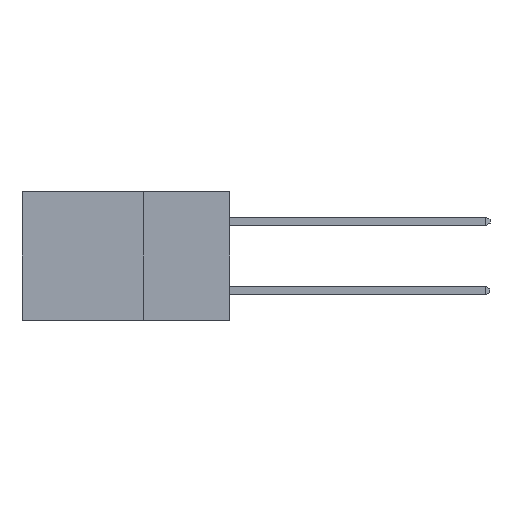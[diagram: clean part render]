
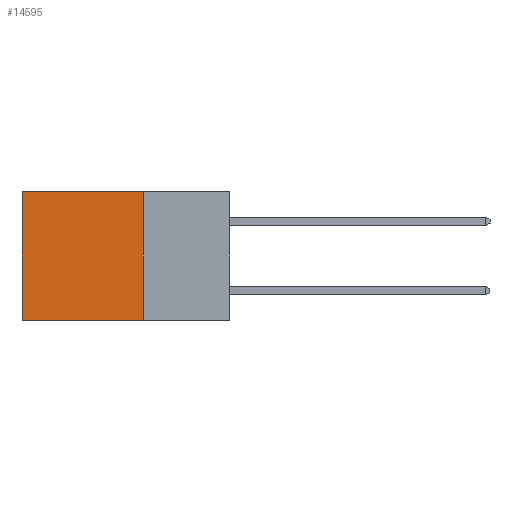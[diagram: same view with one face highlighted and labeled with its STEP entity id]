
A CAD part, left-side view. The second image highlights one B-rep face of the part: STEP entity #14595.
In plain terms, the highlighted planar face has unit normal (-1, 0, 0).
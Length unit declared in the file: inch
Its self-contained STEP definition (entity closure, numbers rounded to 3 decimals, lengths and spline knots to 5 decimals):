
#228 = EDGE_CURVE ( 'NONE', #10772, #3027, #12174, .T. ) ;
#235 = CARTESIAN_POINT ( 'NONE',  ( 0.298, 0.25, 0. ) ) ;
#548 = CARTESIAN_POINT ( 'NONE',  ( 0.298, 0.25, -0.37 ) ) ;
#969 = DIRECTION ( 'NONE',  ( 0., 0., -1. ) ) ;
#998 = EDGE_CURVE ( 'NONE', #12565, #10772, #10539, .T. ) ;
#1278 = LINE ( 'NONE', #548, #7105 ) ;
#1684 = CARTESIAN_POINT ( 'NONE',  ( 0.298, 0.6, 0. ) ) ;
#2713 = DIRECTION ( 'NONE',  ( 1., 0., 0. ) ) ;
#3027 = VERTEX_POINT ( 'NONE', #4455 ) ;
#3034 = CARTESIAN_POINT ( 'NONE',  ( 0.298, 0.6, 0. ) ) ;
#3266 = LINE ( 'NONE', #3469, #9835 ) ;
#3284 = ORIENTED_EDGE ( 'NONE', *, *, #228, .T. ) ;
#3469 = CARTESIAN_POINT ( 'NONE',  ( 0.298, 0.25, 0. ) ) ;
#4455 = CARTESIAN_POINT ( 'NONE',  ( 0.298, 0.6, -0.37 ) ) ;
#4891 = DIRECTION ( 'NONE',  ( 0., 1., 0. ) ) ;
#4924 = EDGE_LOOP ( 'NONE', ( #3284, #9268, #8479, #12929 ) ) ;
#5196 = DIRECTION ( 'NONE',  ( 0., 1., 0. ) ) ;
#6212 = PLANE ( 'NONE',  #14127 ) ;
#7105 = VECTOR ( 'NONE', #5196, 39.37008 ) ;
#7420 = VECTOR ( 'NONE', #4891, 39.37008 ) ;
#7896 = CARTESIAN_POINT ( 'NONE',  ( 0.298, 0.25, -0.37 ) ) ;
#8479 = ORIENTED_EDGE ( 'NONE', *, *, #14366, .F. ) ;
#8539 = DIRECTION ( 'NONE',  ( 0., 0., -1. ) ) ;
#9268 = ORIENTED_EDGE ( 'NONE', *, *, #12765, .F. ) ;
#9835 = VECTOR ( 'NONE', #11619, 39.37008 ) ;
#10539 = LINE ( 'NONE', #13811, #7420 ) ;
#10757 = CARTESIAN_POINT ( 'NONE',  ( 0.298, 0.25, 0. ) ) ;
#10772 = VERTEX_POINT ( 'NONE', #1684 ) ;
#11619 = DIRECTION ( 'NONE',  ( 0., 0., -1. ) ) ;
#11813 = VECTOR ( 'NONE', #969, 39.37008 ) ;
#12174 = LINE ( 'NONE', #3034, #11813 ) ;
#12565 = VERTEX_POINT ( 'NONE', #235 ) ;
#12765 = EDGE_CURVE ( 'NONE', #13626, #3027, #1278, .T. ) ;
#12929 = ORIENTED_EDGE ( 'NONE', *, *, #998, .T. ) ;
#13626 = VERTEX_POINT ( 'NONE', #7896 ) ;
#13811 = CARTESIAN_POINT ( 'NONE',  ( 0.298, 0.25, 0. ) ) ;
#14127 = AXIS2_PLACEMENT_3D ( 'NONE', #10757, #2713, #8539 ) ;
#14366 = EDGE_CURVE ( 'NONE', #12565, #13626, #3266, .T. ) ;
#14595 = ADVANCED_FACE ( 'NONE', ( #14670 ), #6212, .F. ) ;
#14670 = FACE_OUTER_BOUND ( 'NONE', #4924, .T. ) ;
